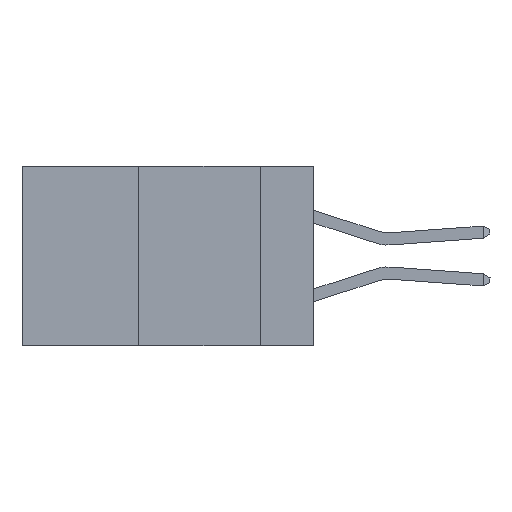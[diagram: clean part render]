
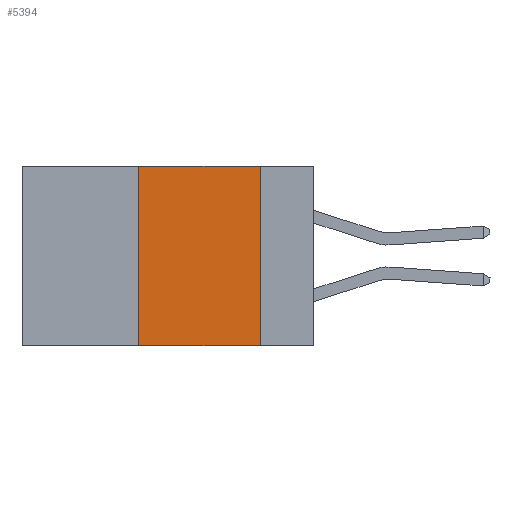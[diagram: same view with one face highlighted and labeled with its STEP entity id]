
A CAD part, left-side view. The second image highlights one B-rep face of the part: STEP entity #5394.
In plain terms, the highlighted planar face has unit normal (-1, 0, 0).
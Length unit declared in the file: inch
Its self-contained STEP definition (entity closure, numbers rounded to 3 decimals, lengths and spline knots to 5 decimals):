
#238 = CARTESIAN_POINT ( 'NONE',  ( 0., 0.36, -0.37 ) ) ;
#486 = EDGE_CURVE ( 'NONE', #1013, #1987, #8748, .T. ) ;
#1013 = VERTEX_POINT ( 'NONE', #238 ) ;
#1073 = CARTESIAN_POINT ( 'NONE',  ( 0., 0.36, 0. ) ) ;
#1078 = DIRECTION ( 'NONE',  ( 1., 0., 0. ) ) ;
#1263 = DIRECTION ( 'NONE',  ( 0., 0., 1. ) ) ;
#1987 = VERTEX_POINT ( 'NONE', #8720 ) ;
#2497 = ORIENTED_EDGE ( 'NONE', *, *, #9606, .F. ) ;
#2501 = EDGE_CURVE ( 'NONE', #1013, #9102, #5352, .T. ) ;
#3581 = LINE ( 'NONE', #5975, #8218 ) ;
#3793 = EDGE_LOOP ( 'NONE', ( #10564, #2497, #10975, #5017 ) ) ;
#3889 = VECTOR ( 'NONE', #9573, 39.37008 ) ;
#4038 = VECTOR ( 'NONE', #4783, 39.37008 ) ;
#4376 = EDGE_CURVE ( 'NONE', #7644, #9102, #3581, .T. ) ;
#4479 = AXIS2_PLACEMENT_3D ( 'NONE', #10207, #1078, #7005 ) ;
#4783 = DIRECTION ( 'NONE',  ( 0., -1., 0. ) ) ;
#5017 = ORIENTED_EDGE ( 'NONE', *, *, #2501, .T. ) ;
#5352 = LINE ( 'NONE', #9631, #3889 ) ;
#5394 = ADVANCED_FACE ( 'NONE', ( #6330 ), #9382, .F. ) ;
#5975 = CARTESIAN_POINT ( 'NONE',  ( 0., 0.11, 0. ) ) ;
#6330 = FACE_OUTER_BOUND ( 'NONE', #3793, .T. ) ;
#6465 = CARTESIAN_POINT ( 'NONE',  ( 0., 0.6, 0. ) ) ;
#7005 = DIRECTION ( 'NONE',  ( 0., 0., -1. ) ) ;
#7644 = VERTEX_POINT ( 'NONE', #9317 ) ;
#8218 = VECTOR ( 'NONE', #8339, 39.37008 ) ;
#8339 = DIRECTION ( 'NONE',  ( 0., 0., -1. ) ) ;
#8355 = CARTESIAN_POINT ( 'NONE',  ( 0., 0.11, -0.37 ) ) ;
#8409 = LINE ( 'NONE', #6465, #4038 ) ;
#8720 = CARTESIAN_POINT ( 'NONE',  ( 0., 0.36, 0. ) ) ;
#8748 = LINE ( 'NONE', #1073, #10644 ) ;
#9102 = VERTEX_POINT ( 'NONE', #8355 ) ;
#9317 = CARTESIAN_POINT ( 'NONE',  ( 0., 0.11, 0. ) ) ;
#9382 = PLANE ( 'NONE',  #4479 ) ;
#9573 = DIRECTION ( 'NONE',  ( 0., -1., 0. ) ) ;
#9606 = EDGE_CURVE ( 'NONE', #1987, #7644, #8409, .T. ) ;
#9631 = CARTESIAN_POINT ( 'NONE',  ( 0., 0.6, -0.37 ) ) ;
#10207 = CARTESIAN_POINT ( 'NONE',  ( 0., 0.6, 0. ) ) ;
#10564 = ORIENTED_EDGE ( 'NONE', *, *, #4376, .F. ) ;
#10644 = VECTOR ( 'NONE', #1263, 39.37008 ) ;
#10975 = ORIENTED_EDGE ( 'NONE', *, *, #486, .F. ) ;
